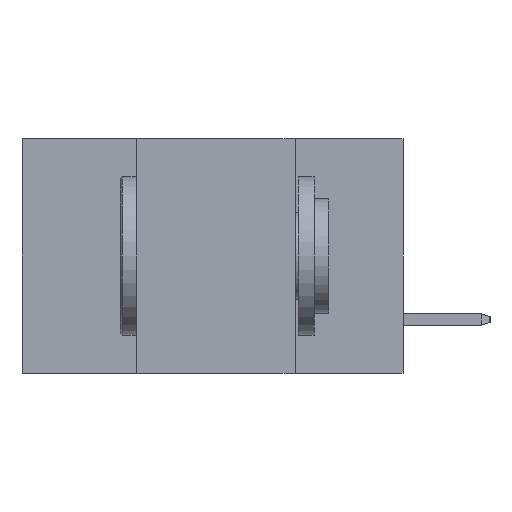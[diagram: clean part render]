
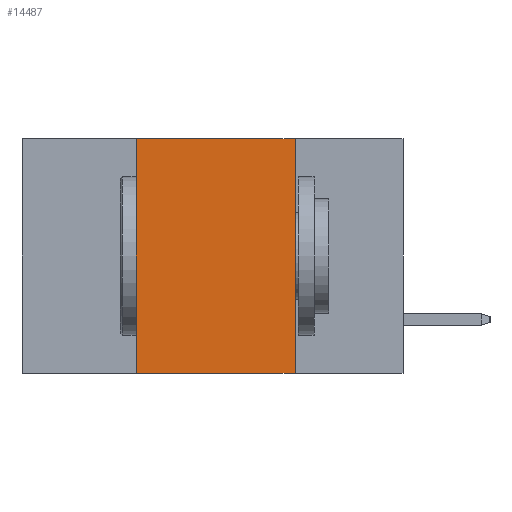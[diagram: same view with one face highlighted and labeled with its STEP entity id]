
A CAD part, left-side view. The second image highlights one B-rep face of the part: STEP entity #14487.
In plain terms, the highlighted planar face has unit normal (-1, 0, 0).
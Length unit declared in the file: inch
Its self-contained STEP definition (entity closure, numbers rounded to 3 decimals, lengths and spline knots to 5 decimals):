
#102 = VECTOR ( 'NONE', #4551, 39.37008 ) ;
#1249 = EDGE_LOOP ( 'NONE', ( #8224, #13613, #8381, #10676 ) ) ;
#1425 = CARTESIAN_POINT ( 'NONE',  ( 0., 0.6, 0. ) ) ;
#1590 = AXIS2_PLACEMENT_3D ( 'NONE', #1425, #14006, #13930 ) ;
#1807 = DIRECTION ( 'NONE',  ( 0., -1., 0. ) ) ;
#1972 = LINE ( 'NONE', #3576, #102 ) ;
#2059 = EDGE_CURVE ( 'NONE', #14778, #5312, #6820, .T. ) ;
#3143 = EDGE_CURVE ( 'NONE', #10872, #16101, #1972, .T. ) ;
#3238 = LINE ( 'NONE', #8361, #12308 ) ;
#3576 = CARTESIAN_POINT ( 'NONE',  ( 0., 0.42, 0. ) ) ;
#3921 = PLANE ( 'NONE',  #1590 ) ;
#4239 = EDGE_CURVE ( 'NONE', #16101, #14778, #3238, .T. ) ;
#4551 = DIRECTION ( 'NONE',  ( 0., 0., 1. ) ) ;
#5137 = VECTOR ( 'NONE', #15778, 39.37008 ) ;
#5312 = VERTEX_POINT ( 'NONE', #7721 ) ;
#5454 = CARTESIAN_POINT ( 'NONE',  ( 0., 0.6, -0.37 ) ) ;
#6820 = LINE ( 'NONE', #15604, #5137 ) ;
#7185 = EDGE_CURVE ( 'NONE', #10872, #5312, #8021, .T. ) ;
#7721 = CARTESIAN_POINT ( 'NONE',  ( 0., 0.17, -0.37 ) ) ;
#8021 = LINE ( 'NONE', #5454, #11808 ) ;
#8224 = ORIENTED_EDGE ( 'NONE', *, *, #2059, .F. ) ;
#8361 = CARTESIAN_POINT ( 'NONE',  ( 0., 0.6, 0. ) ) ;
#8381 = ORIENTED_EDGE ( 'NONE', *, *, #3143, .F. ) ;
#9042 = FACE_OUTER_BOUND ( 'NONE', #1249, .T. ) ;
#10676 = ORIENTED_EDGE ( 'NONE', *, *, #7185, .T. ) ;
#10872 = VERTEX_POINT ( 'NONE', #14485 ) ;
#11808 = VECTOR ( 'NONE', #15557, 39.37008 ) ;
#12308 = VECTOR ( 'NONE', #1807, 39.37008 ) ;
#13241 = CARTESIAN_POINT ( 'NONE',  ( 0., 0.17, 0. ) ) ;
#13613 = ORIENTED_EDGE ( 'NONE', *, *, #4239, .F. ) ;
#13930 = DIRECTION ( 'NONE',  ( 0., 0., -1. ) ) ;
#14006 = DIRECTION ( 'NONE',  ( 1., 0., 0. ) ) ;
#14485 = CARTESIAN_POINT ( 'NONE',  ( 0., 0.42, -0.37 ) ) ;
#14487 = ADVANCED_FACE ( 'NONE', ( #9042 ), #3921, .F. ) ;
#14778 = VERTEX_POINT ( 'NONE', #13241 ) ;
#14921 = CARTESIAN_POINT ( 'NONE',  ( 0., 0.42, 0. ) ) ;
#15557 = DIRECTION ( 'NONE',  ( 0., -1., 0. ) ) ;
#15604 = CARTESIAN_POINT ( 'NONE',  ( 0., 0.17, 0. ) ) ;
#15778 = DIRECTION ( 'NONE',  ( 0., 0., -1. ) ) ;
#16101 = VERTEX_POINT ( 'NONE', #14921 ) ;
